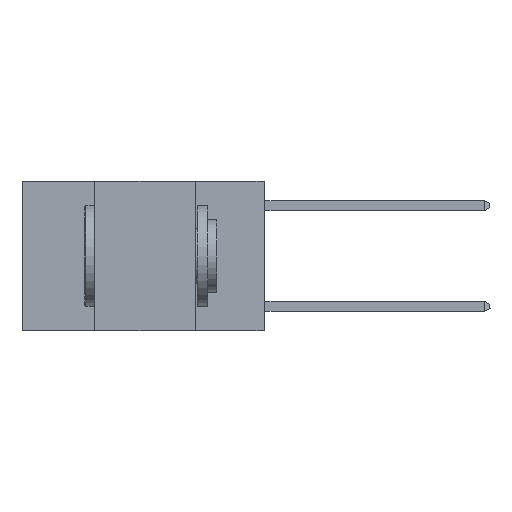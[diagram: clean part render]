
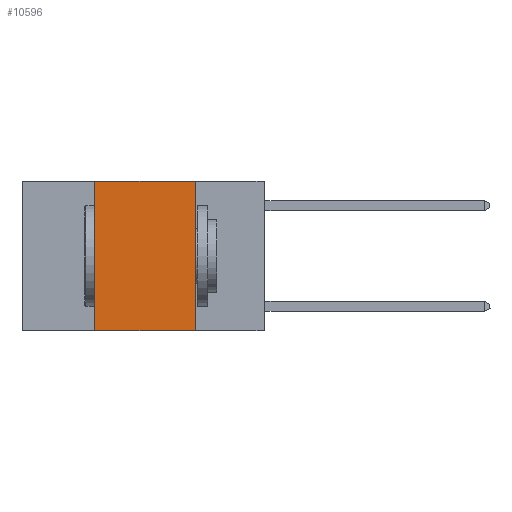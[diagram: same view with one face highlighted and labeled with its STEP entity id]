
A CAD part, left-side view. The second image highlights one B-rep face of the part: STEP entity #10596.
In plain terms, the highlighted planar face has unit normal (-1, 0, 0).
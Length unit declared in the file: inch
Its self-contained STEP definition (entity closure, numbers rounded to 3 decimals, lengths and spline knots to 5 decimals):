
#331 = LINE ( 'NONE', #2853, #12811 ) ;
#556 = EDGE_LOOP ( 'NONE', ( #9785, #2934, #1046, #10181 ) ) ;
#814 = EDGE_CURVE ( 'NONE', #7006, #4538, #4747, .T. ) ;
#1046 = ORIENTED_EDGE ( 'NONE', *, *, #5929, .F. ) ;
#1103 = DIRECTION ( 'NONE',  ( 1., 0., 0. ) ) ;
#1896 = CARTESIAN_POINT ( 'NONE',  ( 0., 0.42, 0. ) ) ;
#2853 = CARTESIAN_POINT ( 'NONE',  ( 0., 0.42, 0. ) ) ;
#2934 = ORIENTED_EDGE ( 'NONE', *, *, #814, .F. ) ;
#3498 = VECTOR ( 'NONE', #14173, 39.37008 ) ;
#4353 = AXIS2_PLACEMENT_3D ( 'NONE', #6902, #1103, #14018 ) ;
#4484 = CARTESIAN_POINT ( 'NONE',  ( 0., 0.17, 0. ) ) ;
#4538 = VERTEX_POINT ( 'NONE', #6265 ) ;
#4747 = LINE ( 'NONE', #9434, #5112 ) ;
#5055 = CARTESIAN_POINT ( 'NONE',  ( 0., 0.42, -0.37 ) ) ;
#5112 = VECTOR ( 'NONE', #5997, 39.37008 ) ;
#5787 = EDGE_CURVE ( 'NONE', #5981, #6075, #9488, .T. ) ;
#5929 = EDGE_CURVE ( 'NONE', #5981, #7006, #331, .T. ) ;
#5981 = VERTEX_POINT ( 'NONE', #5055 ) ;
#5997 = DIRECTION ( 'NONE',  ( 0., -1., 0. ) ) ;
#6075 = VERTEX_POINT ( 'NONE', #8929 ) ;
#6265 = CARTESIAN_POINT ( 'NONE',  ( 0., 0.17, 0. ) ) ;
#6902 = CARTESIAN_POINT ( 'NONE',  ( 0., 0.6, 0. ) ) ;
#6967 = LINE ( 'NONE', #4484, #12246 ) ;
#7006 = VERTEX_POINT ( 'NONE', #1896 ) ;
#7030 = FACE_OUTER_BOUND ( 'NONE', #556, .T. ) ;
#7502 = DIRECTION ( 'NONE',  ( 0., 0., 1. ) ) ;
#8929 = CARTESIAN_POINT ( 'NONE',  ( 0., 0.17, -0.37 ) ) ;
#9434 = CARTESIAN_POINT ( 'NONE',  ( 0., 0.6, 0. ) ) ;
#9488 = LINE ( 'NONE', #13822, #3498 ) ;
#9785 = ORIENTED_EDGE ( 'NONE', *, *, #12523, .F. ) ;
#10181 = ORIENTED_EDGE ( 'NONE', *, *, #5787, .T. ) ;
#10596 = ADVANCED_FACE ( 'NONE', ( #7030 ), #11685, .F. ) ;
#11685 = PLANE ( 'NONE',  #4353 ) ;
#12246 = VECTOR ( 'NONE', #15088, 39.37008 ) ;
#12523 = EDGE_CURVE ( 'NONE', #4538, #6075, #6967, .T. ) ;
#12811 = VECTOR ( 'NONE', #7502, 39.37008 ) ;
#13822 = CARTESIAN_POINT ( 'NONE',  ( 0., 0.6, -0.37 ) ) ;
#14018 = DIRECTION ( 'NONE',  ( 0., 0., -1. ) ) ;
#14173 = DIRECTION ( 'NONE',  ( 0., -1., 0. ) ) ;
#15088 = DIRECTION ( 'NONE',  ( 0., 0., -1. ) ) ;
